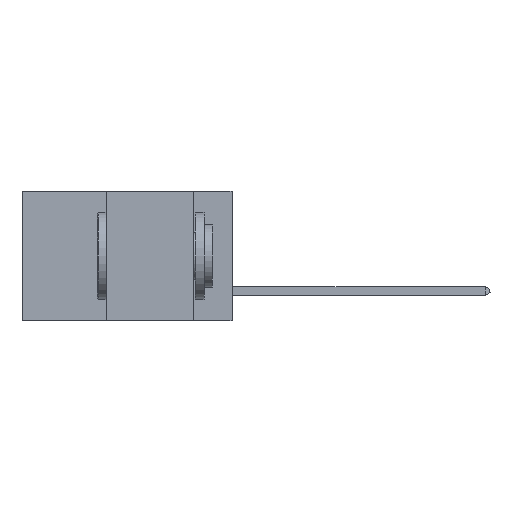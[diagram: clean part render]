
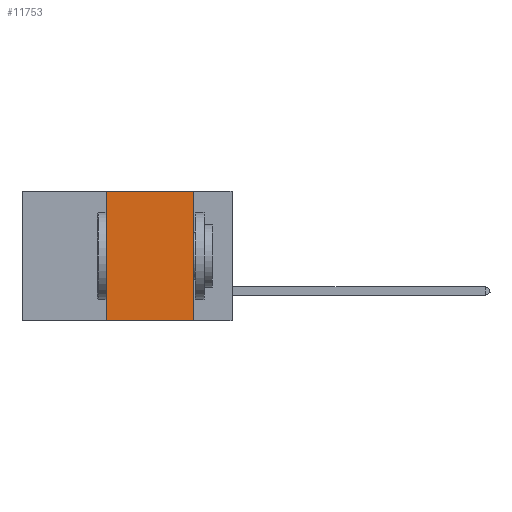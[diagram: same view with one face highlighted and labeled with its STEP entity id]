
A CAD part, left-side view. The second image highlights one B-rep face of the part: STEP entity #11753.
In plain terms, the highlighted planar face has unit normal (-1, 0, 0).
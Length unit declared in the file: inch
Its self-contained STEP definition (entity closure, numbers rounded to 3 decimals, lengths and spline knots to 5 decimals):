
#857 = ORIENTED_EDGE ( 'NONE', *, *, #24524, .F. ) ;
#1034 = PLANE ( 'NONE',  #30064 ) ;
#4249 = CARTESIAN_POINT ( 'NONE',  ( 0., 0.36, 0. ) ) ;
#5306 = EDGE_CURVE ( 'NONE', #15952, #23083, #14830, .T. ) ;
#7958 = VECTOR ( 'NONE', #33011, 39.37008 ) ;
#9882 = EDGE_LOOP ( 'NONE', ( #27293, #857, #27547, #17662 ) ) ;
#10087 = LINE ( 'NONE', #17114, #27670 ) ;
#10862 = CARTESIAN_POINT ( 'NONE',  ( 0., 0.11, -0.37 ) ) ;
#11337 = CARTESIAN_POINT ( 'NONE',  ( 0., 0.6, -0.37 ) ) ;
#11753 = ADVANCED_FACE ( 'NONE', ( #20208 ), #1034, .F. ) ;
#12650 = LINE ( 'NONE', #29782, #7958 ) ;
#14830 = LINE ( 'NONE', #11337, #38004 ) ;
#15952 = VERTEX_POINT ( 'NONE', #18729 ) ;
#17114 = CARTESIAN_POINT ( 'NONE',  ( 0., 0.11, 0. ) ) ;
#17431 = VERTEX_POINT ( 'NONE', #29319 ) ;
#17662 = ORIENTED_EDGE ( 'NONE', *, *, #5306, .T. ) ;
#18729 = CARTESIAN_POINT ( 'NONE',  ( 0., 0.36, -0.37 ) ) ;
#19035 = DIRECTION ( 'NONE',  ( 1., 0., 0. ) ) ;
#20208 = FACE_OUTER_BOUND ( 'NONE', #9882, .T. ) ;
#22650 = EDGE_CURVE ( 'NONE', #17431, #23083, #10087, .T. ) ;
#23083 = VERTEX_POINT ( 'NONE', #10862 ) ;
#23324 = VECTOR ( 'NONE', #30518, 39.37008 ) ;
#24524 = EDGE_CURVE ( 'NONE', #34773, #17431, #25629, .T. ) ;
#24718 = CARTESIAN_POINT ( 'NONE',  ( 0., 0.6, 0. ) ) ;
#25629 = LINE ( 'NONE', #30401, #23324 ) ;
#27293 = ORIENTED_EDGE ( 'NONE', *, *, #22650, .F. ) ;
#27547 = ORIENTED_EDGE ( 'NONE', *, *, #34520, .F. ) ;
#27670 = VECTOR ( 'NONE', #29036, 39.37008 ) ;
#29036 = DIRECTION ( 'NONE',  ( 0., 0., -1. ) ) ;
#29319 = CARTESIAN_POINT ( 'NONE',  ( 0., 0.11, 0. ) ) ;
#29782 = CARTESIAN_POINT ( 'NONE',  ( 0., 0.36, 0. ) ) ;
#30064 = AXIS2_PLACEMENT_3D ( 'NONE', #24718, #19035, #30943 ) ;
#30401 = CARTESIAN_POINT ( 'NONE',  ( 0., 0.6, 0. ) ) ;
#30518 = DIRECTION ( 'NONE',  ( 0., -1., 0. ) ) ;
#30943 = DIRECTION ( 'NONE',  ( 0., 0., -1. ) ) ;
#33011 = DIRECTION ( 'NONE',  ( 0., 0., 1. ) ) ;
#34197 = DIRECTION ( 'NONE',  ( 0., -1., 0. ) ) ;
#34520 = EDGE_CURVE ( 'NONE', #15952, #34773, #12650, .T. ) ;
#34773 = VERTEX_POINT ( 'NONE', #4249 ) ;
#38004 = VECTOR ( 'NONE', #34197, 39.37008 ) ;
